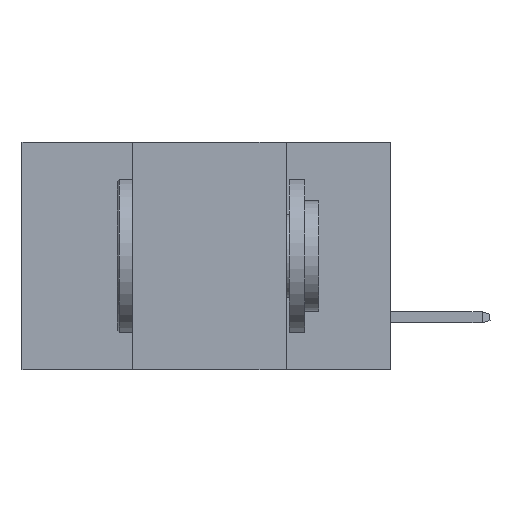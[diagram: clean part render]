
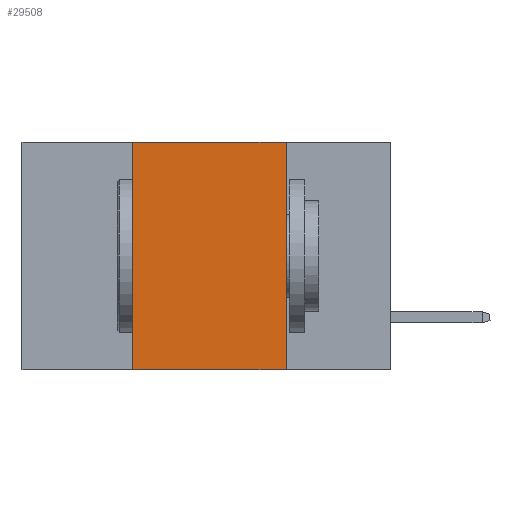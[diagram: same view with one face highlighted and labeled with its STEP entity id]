
A CAD part, left-side view. The second image highlights one B-rep face of the part: STEP entity #29508.
In plain terms, the highlighted planar face has unit normal (-1, 0, 0).
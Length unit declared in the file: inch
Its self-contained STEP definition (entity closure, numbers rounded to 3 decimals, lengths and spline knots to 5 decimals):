
#479 = LINE ( 'NONE', #20111, #12380 ) ;
#521 = LINE ( 'NONE', #20813, #17885 ) ;
#864 = CARTESIAN_POINT ( 'NONE',  ( 0., 0.17, 0. ) ) ;
#1688 = AXIS2_PLACEMENT_3D ( 'NONE', #29621, #16131, #1901 ) ;
#1901 = DIRECTION ( 'NONE',  ( 0., 0., -1. ) ) ;
#3349 = VECTOR ( 'NONE', #22554, 39.37008 ) ;
#6273 = CARTESIAN_POINT ( 'NONE',  ( 0., 0.42, 0. ) ) ;
#7460 = EDGE_CURVE ( 'NONE', #25981, #25317, #15993, .T. ) ;
#7611 = FACE_OUTER_BOUND ( 'NONE', #24498, .T. ) ;
#7683 = VECTOR ( 'NONE', #9117, 39.37008 ) ;
#7854 = CARTESIAN_POINT ( 'NONE',  ( 0., 0.17, -0.37 ) ) ;
#9117 = DIRECTION ( 'NONE',  ( 0., -1., 0. ) ) ;
#9359 = VERTEX_POINT ( 'NONE', #7854 ) ;
#10925 = ORIENTED_EDGE ( 'NONE', *, *, #17793, .F. ) ;
#12380 = VECTOR ( 'NONE', #22452, 39.37008 ) ;
#12398 = ORIENTED_EDGE ( 'NONE', *, *, #29573, .F. ) ;
#14001 = LINE ( 'NONE', #25254, #7683 ) ;
#14560 = CARTESIAN_POINT ( 'NONE',  ( 0., 0.42, -0.37 ) ) ;
#15393 = EDGE_CURVE ( 'NONE', #25981, #9359, #14001, .T. ) ;
#15993 = LINE ( 'NONE', #6273, #3349 ) ;
#16131 = DIRECTION ( 'NONE',  ( 1., 0., 0. ) ) ;
#16825 = CARTESIAN_POINT ( 'NONE',  ( 0., 0.42, 0. ) ) ;
#17793 = EDGE_CURVE ( 'NONE', #25317, #27473, #479, .T. ) ;
#17885 = VECTOR ( 'NONE', #29814, 39.37008 ) ;
#18318 = PLANE ( 'NONE',  #1688 ) ;
#20111 = CARTESIAN_POINT ( 'NONE',  ( 0., 0.6, 0. ) ) ;
#20813 = CARTESIAN_POINT ( 'NONE',  ( 0., 0.17, 0. ) ) ;
#21079 = ORIENTED_EDGE ( 'NONE', *, *, #15393, .T. ) ;
#21790 = ORIENTED_EDGE ( 'NONE', *, *, #7460, .F. ) ;
#22452 = DIRECTION ( 'NONE',  ( 0., -1., 0. ) ) ;
#22554 = DIRECTION ( 'NONE',  ( 0., 0., 1. ) ) ;
#24498 = EDGE_LOOP ( 'NONE', ( #12398, #10925, #21790, #21079 ) ) ;
#25254 = CARTESIAN_POINT ( 'NONE',  ( 0., 0.6, -0.37 ) ) ;
#25317 = VERTEX_POINT ( 'NONE', #16825 ) ;
#25981 = VERTEX_POINT ( 'NONE', #14560 ) ;
#27473 = VERTEX_POINT ( 'NONE', #864 ) ;
#29508 = ADVANCED_FACE ( 'NONE', ( #7611 ), #18318, .F. ) ;
#29573 = EDGE_CURVE ( 'NONE', #27473, #9359, #521, .T. ) ;
#29621 = CARTESIAN_POINT ( 'NONE',  ( 0., 0.6, 0. ) ) ;
#29814 = DIRECTION ( 'NONE',  ( 0., 0., -1. ) ) ;
